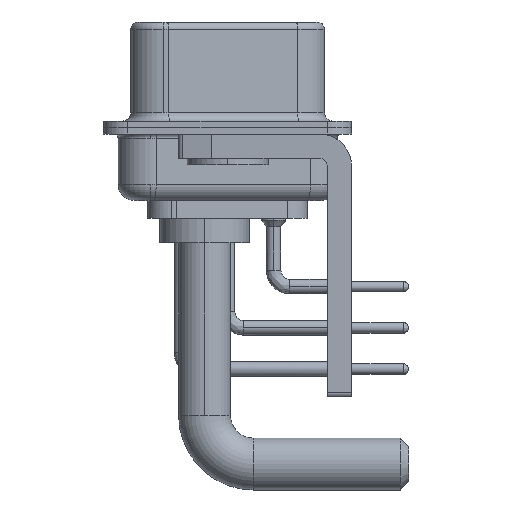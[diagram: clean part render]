
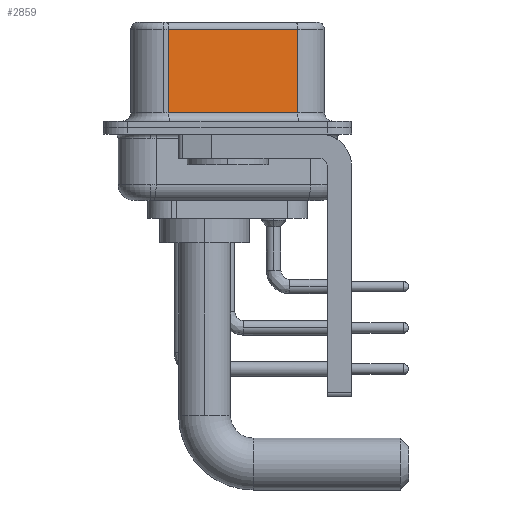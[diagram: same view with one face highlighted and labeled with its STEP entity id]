
A CAD part, left-side view. The second image highlights one B-rep face of the part: STEP entity #2859.
In plain terms, the highlighted planar face has unit normal (-0.985, -0.174, 0).
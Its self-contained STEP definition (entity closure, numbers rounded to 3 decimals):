
#1184 = ORIENTED_EDGE ( 'NONE', *, *, #11654, .T. ) ;
#1200 = DIRECTION ( 'NONE',  ( -0.174, 0.985, 0. ) ) ;
#1578 = DIRECTION ( 'NONE',  ( 0.985, 0.174, 0. ) ) ;
#2859 = ADVANCED_FACE ( 'NONE', ( #4572 ), #26324, .F. ) ;
#3858 = VECTOR ( 'NONE', #16103, 1000. ) ;
#4185 = VECTOR ( 'NONE', #1200, 1000. ) ;
#4572 = FACE_OUTER_BOUND ( 'NONE', #6709, .T. ) ;
#5303 = CARTESIAN_POINT ( 'NONE',  ( 3.73, 3.628, 6.52 ) ) ;
#6686 = LINE ( 'NONE', #25432, #4185 ) ;
#6709 = EDGE_LOOP ( 'NONE', ( #18381, #28965, #1184, #16453 ) ) ;
#6715 = EDGE_CURVE ( 'NONE', #26035, #34901, #13540, .T. ) ;
#11587 = LINE ( 'NONE', #24317, #31418 ) ;
#11654 = EDGE_CURVE ( 'NONE', #28874, #26035, #20882, .T. ) ;
#13540 = LINE ( 'NONE', #32980, #28492 ) ;
#16103 = DIRECTION ( 'NONE',  ( 0., 0., -1. ) ) ;
#16453 = ORIENTED_EDGE ( 'NONE', *, *, #6715, .T. ) ;
#18377 = CARTESIAN_POINT ( 'NONE',  ( 5.132, -4.322, 6.52 ) ) ;
#18381 = ORIENTED_EDGE ( 'NONE', *, *, #24881, .F. ) ;
#20341 = VERTEX_POINT ( 'NONE', #26718 ) ;
#20680 = DIRECTION ( 'NONE',  ( -0.174, 0.985, 0. ) ) ;
#20882 = LINE ( 'NONE', #5303, #3858 ) ;
#21050 = EDGE_CURVE ( 'NONE', #20341, #28874, #6686, .T. ) ;
#22374 = DIRECTION ( 'NONE',  ( 0., 0., -1. ) ) ;
#24317 = CARTESIAN_POINT ( 'NONE',  ( 5.132, -4.322, 6.52 ) ) ;
#24881 = EDGE_CURVE ( 'NONE', #20341, #34901, #11587, .T. ) ;
#25432 = CARTESIAN_POINT ( 'NONE',  ( 5.132, -4.322, 6.02 ) ) ;
#26035 = VERTEX_POINT ( 'NONE', #29304 ) ;
#26166 = AXIS2_PLACEMENT_3D ( 'NONE', #18377, #1578, #20680 ) ;
#26324 = PLANE ( 'NONE',  #26166 ) ;
#26718 = CARTESIAN_POINT ( 'NONE',  ( 5.132, -4.322, 6.02 ) ) ;
#28492 = VECTOR ( 'NONE', #29803, 1000. ) ;
#28874 = VERTEX_POINT ( 'NONE', #31419 ) ;
#28965 = ORIENTED_EDGE ( 'NONE', *, *, #21050, .T. ) ;
#29304 = CARTESIAN_POINT ( 'NONE',  ( 3.73, 3.628, 0.9 ) ) ;
#29803 = DIRECTION ( 'NONE',  ( 0.174, -0.985, 0. ) ) ;
#31418 = VECTOR ( 'NONE', #22374, 1000. ) ;
#31419 = CARTESIAN_POINT ( 'NONE',  ( 3.73, 3.628, 6.02 ) ) ;
#32980 = CARTESIAN_POINT ( 'NONE',  ( 5.132, -4.322, 0.9 ) ) ;
#34350 = CARTESIAN_POINT ( 'NONE',  ( 5.132, -4.322, 0.9 ) ) ;
#34901 = VERTEX_POINT ( 'NONE', #34350 ) ;
